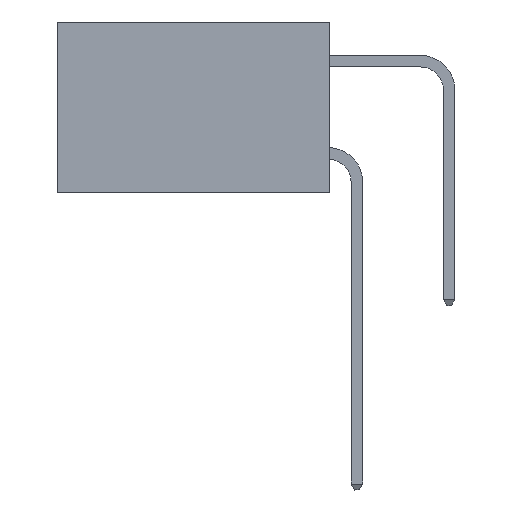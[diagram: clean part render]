
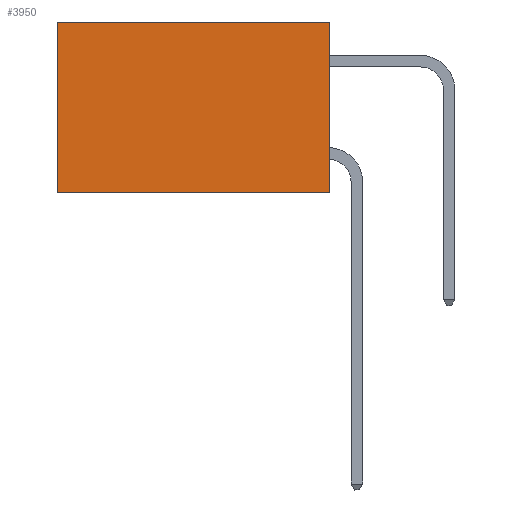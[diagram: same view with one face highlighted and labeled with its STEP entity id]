
A CAD part, left-side view. The second image highlights one B-rep face of the part: STEP entity #3950.
In plain terms, the highlighted planar face has unit normal (-1, 0, 0).
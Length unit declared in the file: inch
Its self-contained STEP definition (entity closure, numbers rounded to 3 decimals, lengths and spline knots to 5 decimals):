
#261 = EDGE_CURVE ( 'NONE', #3610, #535, #3111, .T. ) ;
#535 = VERTEX_POINT ( 'NONE', #10843 ) ;
#1099 = ORIENTED_EDGE ( 'NONE', *, *, #13188, .F. ) ;
#1164 = VECTOR ( 'NONE', #11915, 39.37008 ) ;
#1530 = DIRECTION ( 'NONE',  ( 0., 1., 0. ) ) ;
#1561 = ORIENTED_EDGE ( 'NONE', *, *, #261, .T. ) ;
#1898 = CARTESIAN_POINT ( 'NONE',  ( 0.277, 0.59, -0.37 ) ) ;
#2470 = CARTESIAN_POINT ( 'NONE',  ( 0.277, 0.59, -0.37 ) ) ;
#2594 = CARTESIAN_POINT ( 'NONE',  ( 0.277, 0., -0.37 ) ) ;
#3111 = LINE ( 'NONE', #13852, #17109 ) ;
#3610 = VERTEX_POINT ( 'NONE', #5462 ) ;
#3732 = CARTESIAN_POINT ( 'NONE',  ( 0.277, 0., -0.37 ) ) ;
#3950 = ADVANCED_FACE ( 'NONE', ( #5963 ), #6768, .F. ) ;
#4958 = VERTEX_POINT ( 'NONE', #2594 ) ;
#5166 = EDGE_CURVE ( 'NONE', #535, #8763, #12326, .T. ) ;
#5168 = DIRECTION ( 'NONE',  ( 0., 0., -1. ) ) ;
#5462 = CARTESIAN_POINT ( 'NONE',  ( 0.277, 0., 0. ) ) ;
#5963 = FACE_OUTER_BOUND ( 'NONE', #17403, .T. ) ;
#6626 = DIRECTION ( 'NONE',  ( 0., 0., -1. ) ) ;
#6672 = DIRECTION ( 'NONE',  ( 1., 0., 0. ) ) ;
#6768 = PLANE ( 'NONE',  #10151 ) ;
#7076 = CARTESIAN_POINT ( 'NONE',  ( 0.277, 0., -0.37 ) ) ;
#7404 = VECTOR ( 'NONE', #5168, 39.37008 ) ;
#8763 = VERTEX_POINT ( 'NONE', #1898 ) ;
#10151 = AXIS2_PLACEMENT_3D ( 'NONE', #7076, #6672, #6626 ) ;
#10556 = CARTESIAN_POINT ( 'NONE',  ( 0.277, 0., -0.37 ) ) ;
#10843 = CARTESIAN_POINT ( 'NONE',  ( 0.277, 0.59, 0. ) ) ;
#11570 = ORIENTED_EDGE ( 'NONE', *, *, #5166, .T. ) ;
#11915 = DIRECTION ( 'NONE',  ( 0., 1., 0. ) ) ;
#12326 = LINE ( 'NONE', #2470, #15620 ) ;
#12473 = LINE ( 'NONE', #10556, #1164 ) ;
#13188 = EDGE_CURVE ( 'NONE', #3610, #4958, #14876, .T. ) ;
#13852 = CARTESIAN_POINT ( 'NONE',  ( 0.277, 0., 0. ) ) ;
#14876 = LINE ( 'NONE', #3732, #7404 ) ;
#15620 = VECTOR ( 'NONE', #15626, 39.37008 ) ;
#15626 = DIRECTION ( 'NONE',  ( 0., 0., -1. ) ) ;
#15706 = ORIENTED_EDGE ( 'NONE', *, *, #15983, .F. ) ;
#15983 = EDGE_CURVE ( 'NONE', #4958, #8763, #12473, .T. ) ;
#17109 = VECTOR ( 'NONE', #1530, 39.37008 ) ;
#17403 = EDGE_LOOP ( 'NONE', ( #11570, #15706, #1099, #1561 ) ) ;
